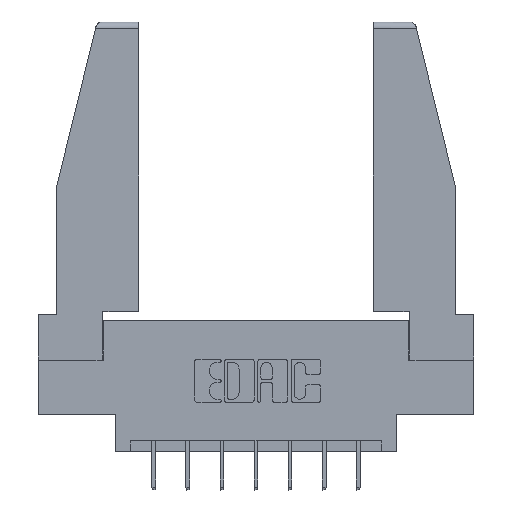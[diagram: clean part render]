
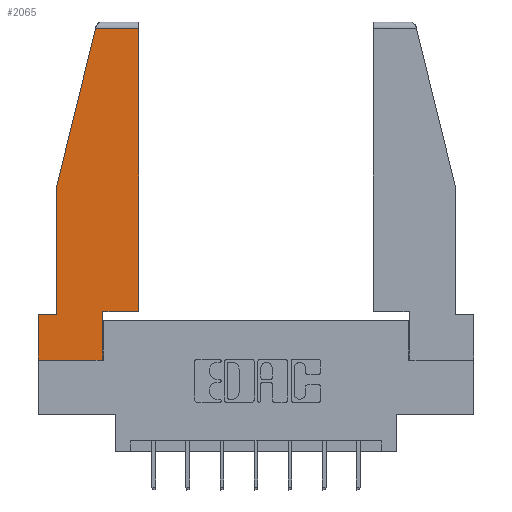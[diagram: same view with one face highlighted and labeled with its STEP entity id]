
A CAD part, top view. The second image highlights one B-rep face of the part: STEP entity #2065.
In plain terms, the highlighted planar face has unit normal (0, 0, 1).
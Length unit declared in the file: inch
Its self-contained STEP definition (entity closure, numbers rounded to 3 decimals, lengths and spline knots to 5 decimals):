
#19 = ORIENTED_EDGE ( 'NONE', *, *, #2078, .T. ) ;
#213 = CARTESIAN_POINT ( 'NONE',  ( 0., 0.21, 0. ) ) ;
#326 = DIRECTION ( 'NONE',  ( -0.239, -0.971, 0. ) ) ;
#411 = CARTESIAN_POINT ( 'NONE',  ( 0., 0., 0. ) ) ;
#434 = VECTOR ( 'NONE', #1666, 39.37008 ) ;
#585 = LINE ( 'NONE', #9207, #5906 ) ;
#707 = VERTEX_POINT ( 'NONE', #3100 ) ;
#905 = ORIENTED_EDGE ( 'NONE', *, *, #7170, .T. ) ;
#1176 = VERTEX_POINT ( 'NONE', #7641 ) ;
#1288 = VERTEX_POINT ( 'NONE', #10845 ) ;
#1396 = DIRECTION ( 'NONE',  ( 1., 0., 0. ) ) ;
#1456 = LINE ( 'NONE', #1477, #9999 ) ;
#1477 = CARTESIAN_POINT ( 'NONE',  ( 0.297, 0., 0. ) ) ;
#1482 = ORIENTED_EDGE ( 'NONE', *, *, #2021, .T. ) ;
#1644 = CARTESIAN_POINT ( 'NONE',  ( 0.297, 0.223, 0. ) ) ;
#1666 = DIRECTION ( 'NONE',  ( 1., 0., 0. ) ) ;
#2021 = EDGE_CURVE ( 'NONE', #2141, #1288, #3161, .T. ) ;
#2065 = ADVANCED_FACE ( 'NONE', ( #12455 ), #5256, .T. ) ;
#2078 = EDGE_CURVE ( 'NONE', #1288, #1176, #585, .T. ) ;
#2141 = VERTEX_POINT ( 'NONE', #11507 ) ;
#2372 = ORIENTED_EDGE ( 'NONE', *, *, #7258, .T. ) ;
#2955 = CARTESIAN_POINT ( 'NONE',  ( 0.461, 0.223, 0. ) ) ;
#3100 = CARTESIAN_POINT ( 'NONE',  ( 0.297, 0.223, 0. ) ) ;
#3153 = AXIS2_PLACEMENT_3D ( 'NONE', #411, #7217, #1396 ) ;
#3161 = LINE ( 'NONE', #8062, #8494 ) ;
#3203 = VERTEX_POINT ( 'NONE', #9588 ) ;
#3225 = CARTESIAN_POINT ( 'NONE',  ( 0.461, 1.52, 0. ) ) ;
#3320 = ORIENTED_EDGE ( 'NONE', *, *, #6838, .T. ) ;
#3387 = DIRECTION ( 'NONE',  ( 0., -1., 0. ) ) ;
#3557 = DIRECTION ( 'NONE',  ( 0., 1., 0. ) ) ;
#3700 = CARTESIAN_POINT ( 'NONE',  ( 0., 0.21, 0. ) ) ;
#3892 = EDGE_CURVE ( 'NONE', #9772, #6817, #7076, .T. ) ;
#4007 = EDGE_CURVE ( 'NONE', #3203, #707, #1456, .T. ) ;
#4086 = ORIENTED_EDGE ( 'NONE', *, *, #4266, .T. ) ;
#4266 = EDGE_CURVE ( 'NONE', #5686, #2141, #6480, .T. ) ;
#5079 = VECTOR ( 'NONE', #11991, 39.37008 ) ;
#5256 = PLANE ( 'NONE',  #3153 ) ;
#5631 = LINE ( 'NONE', #7589, #9462 ) ;
#5686 = VERTEX_POINT ( 'NONE', #3225 ) ;
#5906 = VECTOR ( 'NONE', #3387, 39.37008 ) ;
#6222 = LINE ( 'NONE', #3700, #8200 ) ;
#6480 = LINE ( 'NONE', #6687, #7514 ) ;
#6687 = CARTESIAN_POINT ( 'NONE',  ( 0., 1.52, 0. ) ) ;
#6814 = EDGE_CURVE ( 'NONE', #11657, #5686, #5631, .T. ) ;
#6817 = VERTEX_POINT ( 'NONE', #11582 ) ;
#6838 = EDGE_CURVE ( 'NONE', #707, #11657, #12482, .T. ) ;
#7076 = LINE ( 'NONE', #10095, #5079 ) ;
#7084 = EDGE_LOOP ( 'NONE', ( #8478, #4086, #1482, #19, #2372, #11273, #905, #10297, #3320 ) ) ;
#7170 = EDGE_CURVE ( 'NONE', #6817, #3203, #12605, .T. ) ;
#7217 = DIRECTION ( 'NONE',  ( 0., 0., 1. ) ) ;
#7258 = EDGE_CURVE ( 'NONE', #1176, #9772, #6222, .T. ) ;
#7301 = VECTOR ( 'NONE', #12392, 39.37008 ) ;
#7387 = DIRECTION ( 'NONE',  ( 0., 1., 0. ) ) ;
#7514 = VECTOR ( 'NONE', #11114, 39.37008 ) ;
#7589 = CARTESIAN_POINT ( 'NONE',  ( 0.461, 0.223, 0. ) ) ;
#7641 = CARTESIAN_POINT ( 'NONE',  ( 0.086, 0.21, 0. ) ) ;
#8062 = CARTESIAN_POINT ( 'NONE',  ( 0.271, 1.55, 0. ) ) ;
#8200 = VECTOR ( 'NONE', #11561, 39.37008 ) ;
#8478 = ORIENTED_EDGE ( 'NONE', *, *, #6814, .T. ) ;
#8494 = VECTOR ( 'NONE', #326, 39.37008 ) ;
#9207 = CARTESIAN_POINT ( 'NONE',  ( 0.086, 0.8, 0. ) ) ;
#9462 = VECTOR ( 'NONE', #3557, 39.37008 ) ;
#9588 = CARTESIAN_POINT ( 'NONE',  ( 0.297, 0., 0. ) ) ;
#9772 = VERTEX_POINT ( 'NONE', #213 ) ;
#9999 = VECTOR ( 'NONE', #7387, 39.37008 ) ;
#10095 = CARTESIAN_POINT ( 'NONE',  ( 0., 0.21, 0. ) ) ;
#10297 = ORIENTED_EDGE ( 'NONE', *, *, #4007, .T. ) ;
#10343 = CARTESIAN_POINT ( 'NONE',  ( 0., 0., 0. ) ) ;
#10845 = CARTESIAN_POINT ( 'NONE',  ( 0.086, 0.8, 0. ) ) ;
#11114 = DIRECTION ( 'NONE',  ( -1., 0., 0. ) ) ;
#11273 = ORIENTED_EDGE ( 'NONE', *, *, #3892, .T. ) ;
#11507 = CARTESIAN_POINT ( 'NONE',  ( 0.2636, 1.52, 0. ) ) ;
#11561 = DIRECTION ( 'NONE',  ( -1., 0., 0. ) ) ;
#11582 = CARTESIAN_POINT ( 'NONE',  ( 0., 0., 0. ) ) ;
#11657 = VERTEX_POINT ( 'NONE', #2955 ) ;
#11991 = DIRECTION ( 'NONE',  ( 0., -1., 0. ) ) ;
#12392 = DIRECTION ( 'NONE',  ( 1., 0., 0. ) ) ;
#12455 = FACE_OUTER_BOUND ( 'NONE', #7084, .T. ) ;
#12482 = LINE ( 'NONE', #1644, #7301 ) ;
#12605 = LINE ( 'NONE', #10343, #434 ) ;
